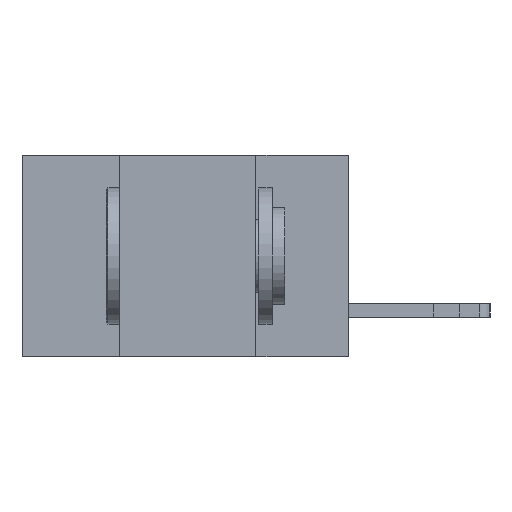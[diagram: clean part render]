
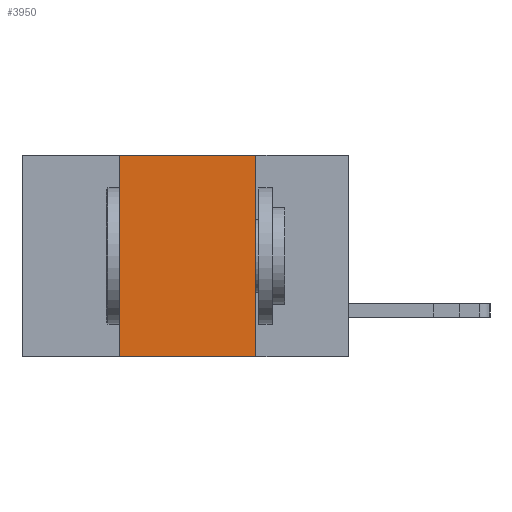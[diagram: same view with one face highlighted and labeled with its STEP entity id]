
A CAD part, left-side view. The second image highlights one B-rep face of the part: STEP entity #3950.
In plain terms, the highlighted planar face has unit normal (-1, 0, 0).
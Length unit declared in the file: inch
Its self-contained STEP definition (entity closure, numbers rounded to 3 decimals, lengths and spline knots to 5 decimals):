
#350 = AXIS2_PLACEMENT_3D ( 'NONE', #3719, #11286, #4885 ) ;
#851 = LINE ( 'NONE', #11020, #6747 ) ;
#1633 = VECTOR ( 'NONE', #7469, 39.37008 ) ;
#2281 = EDGE_LOOP ( 'NONE', ( #7178, #7194, #7205, #7304 ) ) ;
#2816 = VECTOR ( 'NONE', #3996, 39.37008 ) ;
#3188 = LINE ( 'NONE', #5148, #5551 ) ;
#3406 = EDGE_CURVE ( 'NONE', #7889, #7277, #851, .T. ) ;
#3719 = CARTESIAN_POINT ( 'NONE',  ( 0., 0.6, 0. ) ) ;
#3892 = CARTESIAN_POINT ( 'NONE',  ( 0., 0.17, 0. ) ) ;
#3928 = CARTESIAN_POINT ( 'NONE',  ( 0., 0.17, -0.37 ) ) ;
#3950 = ADVANCED_FACE ( 'NONE', ( #13004 ), #10219, .F. ) ;
#3996 = DIRECTION ( 'NONE',  ( 0., -1., 0. ) ) ;
#4859 = LINE ( 'NONE', #6408, #1633 ) ;
#4885 = DIRECTION ( 'NONE',  ( 0., 0., -1. ) ) ;
#4933 = VERTEX_POINT ( 'NONE', #3928 ) ;
#5148 = CARTESIAN_POINT ( 'NONE',  ( 0., 0.42, 0. ) ) ;
#5551 = VECTOR ( 'NONE', #13435, 39.37008 ) ;
#5712 = CARTESIAN_POINT ( 'NONE',  ( 0., 0.42, -0.37 ) ) ;
#6250 = VERTEX_POINT ( 'NONE', #5712 ) ;
#6408 = CARTESIAN_POINT ( 'NONE',  ( 0., 0.17, 0. ) ) ;
#6747 = VECTOR ( 'NONE', #12034, 39.37008 ) ;
#7178 = ORIENTED_EDGE ( 'NONE', *, *, #7490, .F. ) ;
#7194 = ORIENTED_EDGE ( 'NONE', *, *, #3406, .F. ) ;
#7205 = ORIENTED_EDGE ( 'NONE', *, *, #7376, .F. ) ;
#7277 = VERTEX_POINT ( 'NONE', #3892 ) ;
#7304 = ORIENTED_EDGE ( 'NONE', *, *, #7373, .T. ) ;
#7373 = EDGE_CURVE ( 'NONE', #6250, #4933, #11537, .T. ) ;
#7376 = EDGE_CURVE ( 'NONE', #6250, #7889, #3188, .T. ) ;
#7469 = DIRECTION ( 'NONE',  ( 0., 0., -1. ) ) ;
#7490 = EDGE_CURVE ( 'NONE', #7277, #4933, #4859, .T. ) ;
#7889 = VERTEX_POINT ( 'NONE', #10080 ) ;
#10080 = CARTESIAN_POINT ( 'NONE',  ( 0., 0.42, 0. ) ) ;
#10219 = PLANE ( 'NONE',  #350 ) ;
#11020 = CARTESIAN_POINT ( 'NONE',  ( 0., 0.6, 0. ) ) ;
#11286 = DIRECTION ( 'NONE',  ( 1., 0., 0. ) ) ;
#11518 = CARTESIAN_POINT ( 'NONE',  ( 0., 0.6, -0.37 ) ) ;
#11537 = LINE ( 'NONE', #11518, #2816 ) ;
#12034 = DIRECTION ( 'NONE',  ( 0., -1., 0. ) ) ;
#13004 = FACE_OUTER_BOUND ( 'NONE', #2281, .T. ) ;
#13435 = DIRECTION ( 'NONE',  ( 0., 0., 1. ) ) ;
